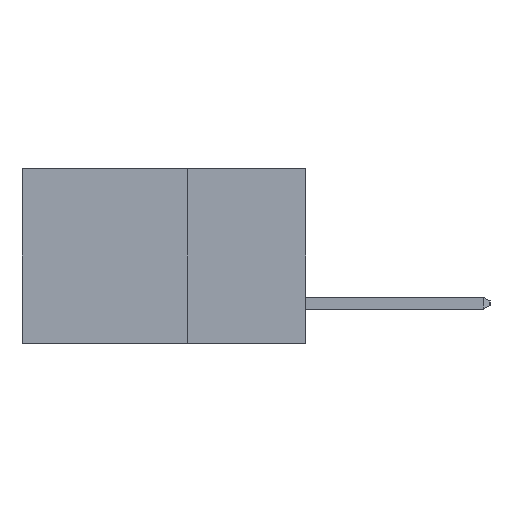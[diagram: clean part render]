
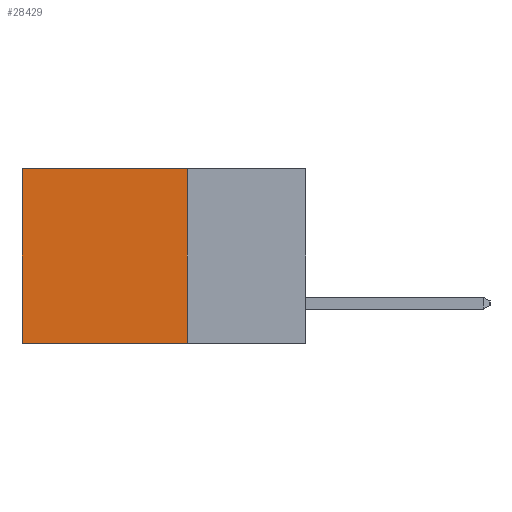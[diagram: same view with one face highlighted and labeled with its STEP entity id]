
A CAD part, left-side view. The second image highlights one B-rep face of the part: STEP entity #28429.
In plain terms, the highlighted planar face has unit normal (-1, 0, 0).
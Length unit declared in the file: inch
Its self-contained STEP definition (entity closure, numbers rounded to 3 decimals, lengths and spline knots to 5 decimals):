
#337 = ORIENTED_EDGE ( 'NONE', *, *, #30271, .T. ) ;
#1131 = ORIENTED_EDGE ( 'NONE', *, *, #12058, .F. ) ;
#2737 = CARTESIAN_POINT ( 'NONE',  ( 0.298, 0.6, -0.37 ) ) ;
#5572 = EDGE_CURVE ( 'NONE', #31143, #13305, #12542, .T. ) ;
#6086 = CARTESIAN_POINT ( 'NONE',  ( 0.298, 0.25, 0. ) ) ;
#6095 = VECTOR ( 'NONE', #10867, 39.37008 ) ;
#6540 = VERTEX_POINT ( 'NONE', #2737 ) ;
#6578 = DIRECTION ( 'NONE',  ( 0., 0., -1. ) ) ;
#7432 = CARTESIAN_POINT ( 'NONE',  ( 0.298, 0.6, 0. ) ) ;
#9226 = DIRECTION ( 'NONE',  ( 0., 1., 0. ) ) ;
#9340 = ORIENTED_EDGE ( 'NONE', *, *, #22050, .T. ) ;
#10867 = DIRECTION ( 'NONE',  ( 0., 0., -1. ) ) ;
#11351 = CARTESIAN_POINT ( 'NONE',  ( 0.298, 0.25, 0. ) ) ;
#11877 = FACE_OUTER_BOUND ( 'NONE', #15866, .T. ) ;
#12058 = EDGE_CURVE ( 'NONE', #13305, #6540, #18935, .T. ) ;
#12542 = LINE ( 'NONE', #22688, #6095 ) ;
#12594 = VECTOR ( 'NONE', #9226, 39.37008 ) ;
#12863 = VERTEX_POINT ( 'NONE', #7432 ) ;
#13305 = VERTEX_POINT ( 'NONE', #25880 ) ;
#13917 = CARTESIAN_POINT ( 'NONE',  ( 0.298, 0.25, -0.37 ) ) ;
#15866 = EDGE_LOOP ( 'NONE', ( #9340, #1131, #19025, #337 ) ) ;
#16184 = PLANE ( 'NONE',  #22837 ) ;
#17105 = CARTESIAN_POINT ( 'NONE',  ( 0.298, 0.25, 0. ) ) ;
#18569 = VECTOR ( 'NONE', #25139, 39.37008 ) ;
#18873 = VECTOR ( 'NONE', #25331, 39.37008 ) ;
#18935 = LINE ( 'NONE', #13917, #12594 ) ;
#19025 = ORIENTED_EDGE ( 'NONE', *, *, #5572, .F. ) ;
#19324 = LINE ( 'NONE', #29996, #18569 ) ;
#20969 = DIRECTION ( 'NONE',  ( 1., 0., 0. ) ) ;
#22050 = EDGE_CURVE ( 'NONE', #12863, #6540, #19324, .T. ) ;
#22688 = CARTESIAN_POINT ( 'NONE',  ( 0.298, 0.25, 0. ) ) ;
#22837 = AXIS2_PLACEMENT_3D ( 'NONE', #11351, #20969, #6578 ) ;
#25139 = DIRECTION ( 'NONE',  ( 0., 0., -1. ) ) ;
#25331 = DIRECTION ( 'NONE',  ( 0., 1., 0. ) ) ;
#25880 = CARTESIAN_POINT ( 'NONE',  ( 0.298, 0.25, -0.37 ) ) ;
#26040 = LINE ( 'NONE', #6086, #18873 ) ;
#28429 = ADVANCED_FACE ( 'NONE', ( #11877 ), #16184, .F. ) ;
#29996 = CARTESIAN_POINT ( 'NONE',  ( 0.298, 0.6, 0. ) ) ;
#30271 = EDGE_CURVE ( 'NONE', #31143, #12863, #26040, .T. ) ;
#31143 = VERTEX_POINT ( 'NONE', #17105 ) ;
